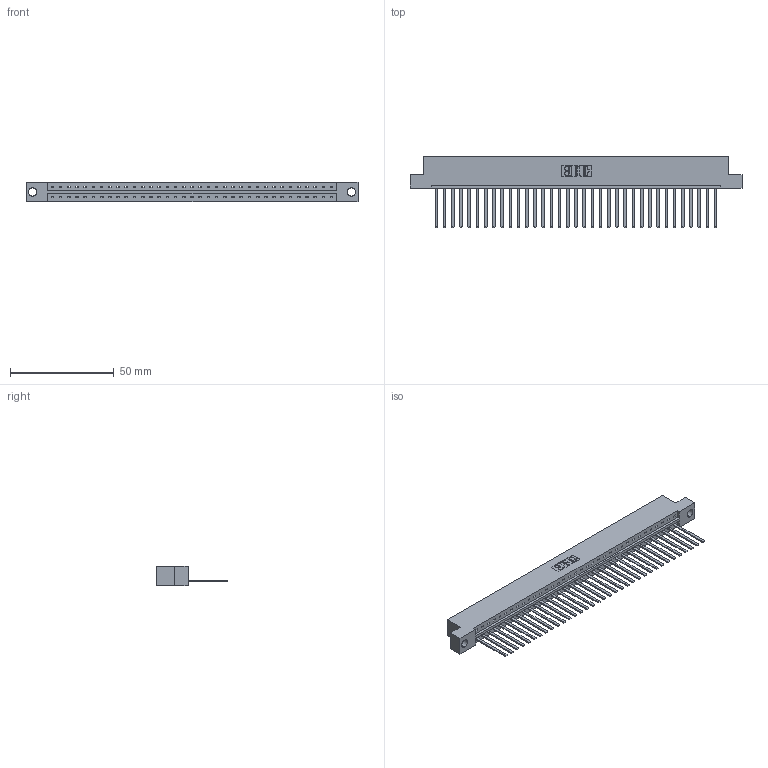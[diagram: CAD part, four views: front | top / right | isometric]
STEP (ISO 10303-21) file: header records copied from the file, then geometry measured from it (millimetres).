
FILE_DESCRIPTION (( 'STEP AP203' ), '1' );
FILE_NAME ('333-035-544-104.STEP', '2018-08-02T23:50:33', ( '' ), ( '' ), 'SwSTEP 2.0', 'SolidWorks 2016', '' );
FILE_SCHEMA (( 'CONFIG_CONTROL_DESIGN' ));
Length unit declared in the file: inch
Products named in the file (3): 333 Part_Flush - .156 Dia - TH; 345-292-001_345-293-144; 333-035-544-104
Assembly tree (36 placements, depth 2):
  333-035-544-104
    333 Part_Flush - .156 Dia - TH
    345-292-001_345-293-144  x35
Bounding box: 160.22 x 34.3 x 9.4 mm (x, y, z)
Volume: 16380.3 mm3; surface area: 18790.8 mm2
Topology: 36 solids, 36 shells, 1934 faces, 5841 edges, 3846 vertices
Faces by surface type: plane 1400, cylinder 534
Entity records: 22121 total; most frequent: CARTESIAN_POINT 3823, ORIENTED_EDGE 3794, DIRECTION 3235, EDGE_CURVE 1897, LINE 1773, VECTOR 1773, VERTEX_POINT 1262, AXIS2_PLACEMENT_3D 731
